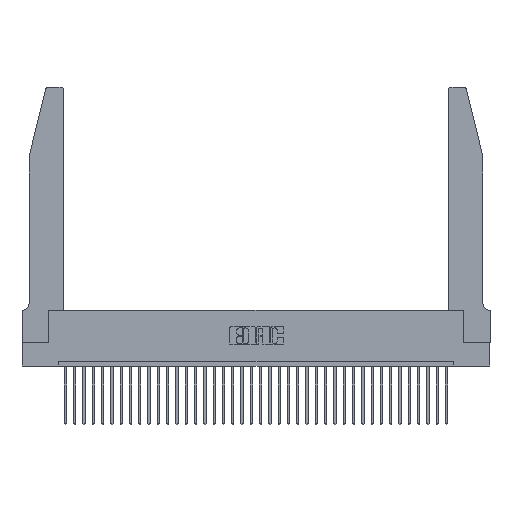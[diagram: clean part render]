
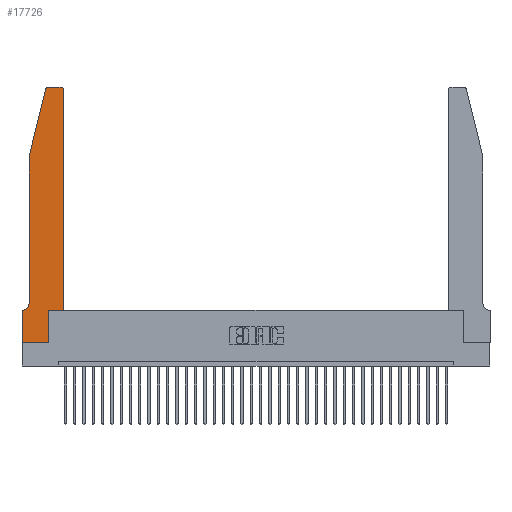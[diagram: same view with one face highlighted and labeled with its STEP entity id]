
A CAD part, top view. The second image highlights one B-rep face of the part: STEP entity #17726.
In plain terms, the highlighted planar face has unit normal (0, 0, 1).
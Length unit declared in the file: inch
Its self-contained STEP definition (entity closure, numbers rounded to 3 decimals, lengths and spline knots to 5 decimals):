
#81 = EDGE_CURVE ( 'NONE', #13681, #14682, #10846, .T. ) ;
#291 = CIRCLE ( 'NONE', #1601, 0.07 ) ;
#582 = CARTESIAN_POINT ( 'NONE',  ( 0.0055, 0.35, 0.37 ) ) ;
#1108 = LINE ( 'NONE', #2088, #9430 ) ;
#1142 = CARTESIAN_POINT ( 'NONE',  ( 0.0755, 0.42, 0.37 ) ) ;
#1601 = AXIS2_PLACEMENT_3D ( 'NONE', #28402, #8191, #16565 ) ;
#1820 = VECTOR ( 'NONE', #15808, 39.37008 ) ;
#1845 = LINE ( 'NONE', #19178, #23850 ) ;
#1914 = EDGE_CURVE ( 'NONE', #29267, #13681, #1108, .T. ) ;
#1997 = CARTESIAN_POINT ( 'NONE',  ( 0.4505, 2.72, 0.37 ) ) ;
#2053 = CARTESIAN_POINT ( 'NONE',  ( 0., 0.35, 0.37 ) ) ;
#2088 = CARTESIAN_POINT ( 'NONE',  ( 0.4505, 0.35, 0.37 ) ) ;
#2235 = CARTESIAN_POINT ( 'NONE',  ( 0.4205, 2.72, 0.37 ) ) ;
#2438 = CARTESIAN_POINT ( 'NONE',  ( 0.0755, 2., 0.37 ) ) ;
#2505 = ORIENTED_EDGE ( 'NONE', *, *, #18215, .T. ) ;
#2556 = DIRECTION ( 'NONE',  ( 1., 0., 0. ) ) ;
#3021 = VERTEX_POINT ( 'NONE', #27347 ) ;
#4491 = ORIENTED_EDGE ( 'NONE', *, *, #9013, .T. ) ;
#4644 = VERTEX_POINT ( 'NONE', #582 ) ;
#4815 = LINE ( 'NONE', #21152, #33869 ) ;
#4843 = DIRECTION ( 'NONE',  ( 1., 0., 0. ) ) ;
#4993 = DIRECTION ( 'NONE',  ( 0., 0., 1. ) ) ;
#5383 = CARTESIAN_POINT ( 'NONE',  ( 0., 0., 0.37 ) ) ;
#5538 = VECTOR ( 'NONE', #17089, 39.37008 ) ;
#5978 = CARTESIAN_POINT ( 'NONE',  ( 0.0755, 2., 0.37 ) ) ;
#6306 = ORIENTED_EDGE ( 'NONE', *, *, #34181, .T. ) ;
#6465 = ORIENTED_EDGE ( 'NONE', *, *, #10492, .T. ) ;
#6939 = CARTESIAN_POINT ( 'NONE',  ( 0.284, 2.72, 0.37 ) ) ;
#7007 = CIRCLE ( 'NONE', #29343, 0.03 ) ;
#7311 = VECTOR ( 'NONE', #23199, 39.37008 ) ;
#8191 = DIRECTION ( 'NONE',  ( 0., 0., -1. ) ) ;
#9013 = EDGE_CURVE ( 'NONE', #26356, #15159, #4815, .T. ) ;
#9430 = VECTOR ( 'NONE', #2556, 39.37008 ) ;
#9736 = CARTESIAN_POINT ( 'NONE',  ( 0.4505, 0.35, 0.37 ) ) ;
#10349 = DIRECTION ( 'NONE',  ( 0., 0., 1. ) ) ;
#10492 = EDGE_CURVE ( 'NONE', #25348, #27765, #14817, .T. ) ;
#10846 = LINE ( 'NONE', #35226, #12224 ) ;
#10863 = LINE ( 'NONE', #5978, #32021 ) ;
#12135 = EDGE_CURVE ( 'NONE', #27765, #16287, #7007, .T. ) ;
#12224 = VECTOR ( 'NONE', #32436, 39.37008 ) ;
#12653 = CARTESIAN_POINT ( 'NONE',  ( 0.2605, 2.75, 0.37 ) ) ;
#13166 = PLANE ( 'NONE',  #36319 ) ;
#13180 = ORIENTED_EDGE ( 'NONE', *, *, #24709, .T. ) ;
#13214 = CIRCLE ( 'NONE', #34200, 0.03 ) ;
#13681 = VERTEX_POINT ( 'NONE', #9736 ) ;
#14682 = VERTEX_POINT ( 'NONE', #1997 ) ;
#14817 = LINE ( 'NONE', #12653, #7311 ) ;
#15035 = EDGE_CURVE ( 'NONE', #3021, #29267, #16470, .T. ) ;
#15159 = VERTEX_POINT ( 'NONE', #19879 ) ;
#15808 = DIRECTION ( 'NONE',  ( -0.239, -0.971, 0. ) ) ;
#16095 = DIRECTION ( 'NONE',  ( -1., 0., 0. ) ) ;
#16287 = VERTEX_POINT ( 'NONE', #32454 ) ;
#16470 = LINE ( 'NONE', #33605, #26195 ) ;
#16565 = DIRECTION ( 'NONE',  ( -1., 0., 0. ) ) ;
#17089 = DIRECTION ( 'NONE',  ( 1., 0., 0. ) ) ;
#17726 = ADVANCED_FACE ( 'NONE', ( #19033 ), #13166, .T. ) ;
#18215 = EDGE_CURVE ( 'NONE', #16287, #29605, #24282, .T. ) ;
#19033 = FACE_OUTER_BOUND ( 'NONE', #21165, .T. ) ;
#19178 = CARTESIAN_POINT ( 'NONE',  ( 0.0755, 0.35, 0.37 ) ) ;
#19879 = CARTESIAN_POINT ( 'NONE',  ( 0., 0., 0.37 ) ) ;
#21152 = CARTESIAN_POINT ( 'NONE',  ( 0., 0., 0.37 ) ) ;
#21165 = EDGE_LOOP ( 'NONE', ( #6465, #26625, #2505, #35073, #13180, #6306, #4491, #25109, #22452, #30649, #22114, #30794 ) ) ;
#21314 = CARTESIAN_POINT ( 'NONE',  ( 0.2865, 0.35, 0.37 ) ) ;
#21595 = CARTESIAN_POINT ( 'NONE',  ( 0.0755, 2., 0.37 ) ) ;
#21769 = EDGE_CURVE ( 'NONE', #15159, #3021, #26734, .T. ) ;
#22106 = DIRECTION ( 'NONE',  ( 1., 0., 0. ) ) ;
#22114 = ORIENTED_EDGE ( 'NONE', *, *, #81, .T. ) ;
#22452 = ORIENTED_EDGE ( 'NONE', *, *, #15035, .T. ) ;
#22744 = DIRECTION ( 'NONE',  ( 0., -1., 0. ) ) ;
#23199 = DIRECTION ( 'NONE',  ( -1., 0., 0. ) ) ;
#23522 = CARTESIAN_POINT ( 'NONE',  ( 0., 0.35, 0.37 ) ) ;
#23850 = VECTOR ( 'NONE', #16095, 39.37008 ) ;
#23980 = DIRECTION ( 'NONE',  ( 0., -1., 0. ) ) ;
#24023 = EDGE_CURVE ( 'NONE', #29605, #28039, #10863, .T. ) ;
#24282 = LINE ( 'NONE', #21595, #1820 ) ;
#24709 = EDGE_CURVE ( 'NONE', #28039, #4644, #291, .T. ) ;
#25109 = ORIENTED_EDGE ( 'NONE', *, *, #21769, .T. ) ;
#25348 = VERTEX_POINT ( 'NONE', #29360 ) ;
#25385 = DIRECTION ( 'NONE',  ( 0., 1., 0. ) ) ;
#26195 = VECTOR ( 'NONE', #25385, 39.37008 ) ;
#26356 = VERTEX_POINT ( 'NONE', #23522 ) ;
#26625 = ORIENTED_EDGE ( 'NONE', *, *, #12135, .T. ) ;
#26734 = LINE ( 'NONE', #5383, #5538 ) ;
#26805 = DIRECTION ( 'NONE',  ( 1., 0., 0. ) ) ;
#27347 = CARTESIAN_POINT ( 'NONE',  ( 0.2865, 0., 0.37 ) ) ;
#27765 = VERTEX_POINT ( 'NONE', #28041 ) ;
#28039 = VERTEX_POINT ( 'NONE', #1142 ) ;
#28041 = CARTESIAN_POINT ( 'NONE',  ( 0.284, 2.75, 0.37 ) ) ;
#28402 = CARTESIAN_POINT ( 'NONE',  ( 0.0055, 0.42, 0.37 ) ) ;
#29267 = VERTEX_POINT ( 'NONE', #21314 ) ;
#29343 = AXIS2_PLACEMENT_3D ( 'NONE', #6939, #32434, #26805 ) ;
#29360 = CARTESIAN_POINT ( 'NONE',  ( 0.4205, 2.75, 0.37 ) ) ;
#29605 = VERTEX_POINT ( 'NONE', #2438 ) ;
#30649 = ORIENTED_EDGE ( 'NONE', *, *, #1914, .T. ) ;
#30794 = ORIENTED_EDGE ( 'NONE', *, *, #35481, .T. ) ;
#32021 = VECTOR ( 'NONE', #22744, 39.37008 ) ;
#32434 = DIRECTION ( 'NONE',  ( 0., 0., 1. ) ) ;
#32436 = DIRECTION ( 'NONE',  ( 0., 1., 0. ) ) ;
#32454 = CARTESIAN_POINT ( 'NONE',  ( 0.25487, 2.72718, 0.37 ) ) ;
#33605 = CARTESIAN_POINT ( 'NONE',  ( 0.2865, 0.35, 0.37 ) ) ;
#33869 = VECTOR ( 'NONE', #23980, 39.37008 ) ;
#34181 = EDGE_CURVE ( 'NONE', #4644, #26356, #1845, .T. ) ;
#34200 = AXIS2_PLACEMENT_3D ( 'NONE', #2235, #10349, #4843 ) ;
#35073 = ORIENTED_EDGE ( 'NONE', *, *, #24023, .T. ) ;
#35226 = CARTESIAN_POINT ( 'NONE',  ( 0.4505, 0.35, 0.37 ) ) ;
#35481 = EDGE_CURVE ( 'NONE', #14682, #25348, #13214, .T. ) ;
#36319 = AXIS2_PLACEMENT_3D ( 'NONE', #2053, #4993, #22106 ) ;
